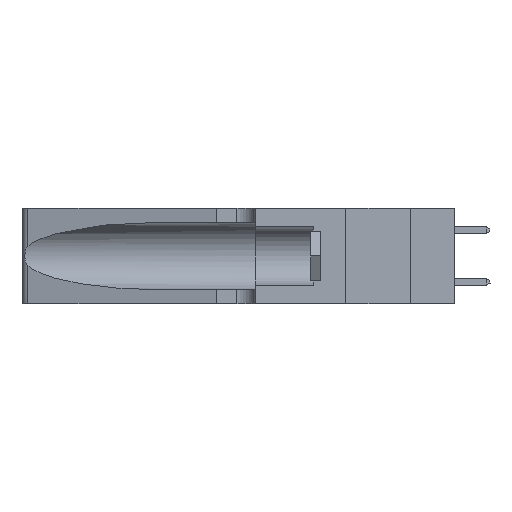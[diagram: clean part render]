
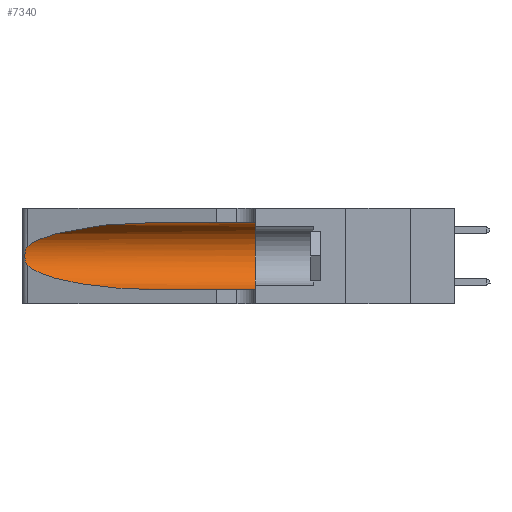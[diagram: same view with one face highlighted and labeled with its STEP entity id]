
A CAD part, left-side view. The second image highlights one B-rep face of the part: STEP entity #7340.
In plain terms, the highlighted cylindrical face has radius 3.308 mm (diameter 6.617 mm), a partial arc.
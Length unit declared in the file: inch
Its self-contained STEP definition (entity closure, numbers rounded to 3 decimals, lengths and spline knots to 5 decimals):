
#622 = CARTESIAN_POINT ( 'NONE',  ( 0.25555, 1.22994, 0.2215 ) ) ;
#775 = CARTESIAN_POINT ( 'NONE',  ( 0.25639, 1.23186, 0.15144 ) ) ;
#1022 = EDGE_CURVE ( 'NONE', #10462, #40487, #26562, .T. ) ;
#1375 = ORIENTED_EDGE ( 'NONE', *, *, #4020, .T. ) ;
#1956 = CARTESIAN_POINT ( 'NONE',  ( 0.2373, 1.15595, 0.28018 ) ) ;
#2164 = CARTESIAN_POINT ( 'NONE',  ( 0.1305, 1.61858, 0.05475 ) ) ;
#3969 = DIRECTION ( 'NONE',  ( 0., 1., 0. ) ) ;
#4020 = EDGE_CURVE ( 'NONE', #10462, #8143, #30314, .T. ) ;
#4248 = CARTESIAN_POINT ( 'NONE',  ( 0.25487, 1.22718, 0.14631 ) ) ;
#4507 = VERTEX_POINT ( 'NONE', #24867 ) ;
#6397 = DIRECTION ( 'NONE',  ( 0., 0., -1. ) ) ;
#6843 = B_SPLINE_CURVE_WITH_KNOTS ( 'NONE', 3,
 ( #24327, #622, #7520, #31050, #10966, #34433, #14373, #37853, #17727, #41245, #21098, #775, #24480, #4248 ),
 .UNSPECIFIED., .F., .F.,
 ( 4, 2, 2, 2, 2, 2, 4 ),
 ( 0., 0.00027, 0.00053, 0.00107, 0.0016, 0.00187, 0.00214 ),
 .UNSPECIFIED. ) ;
#7340 = ADVANCED_FACE ( 'NONE', ( #22718 ), #19573, .F. ) ;
#7520 = CARTESIAN_POINT ( 'NONE',  ( 0.25639, 1.23184, 0.21858 ) ) ;
#8143 = VERTEX_POINT ( 'NONE', #14239 ) ;
#9499 = EDGE_CURVE ( 'NONE', #40487, #18419, #14676, .T. ) ;
#10462 = VERTEX_POINT ( 'NONE', #15334 ) ;
#10966 = CARTESIAN_POINT ( 'NONE',  ( 0.25854, 1.2359, 0.20912 ) ) ;
#11624 = EDGE_CURVE ( 'NONE', #8143, #4507, #6843, .T. ) ;
#12031 = ORIENTED_EDGE ( 'NONE', *, *, #34975, .T. ) ;
#13264 = DIRECTION ( 'NONE',  ( 0., -1., 0. ) ) ;
#14239 = CARTESIAN_POINT ( 'NONE',  ( 0.25487, 1.22718, 0.22369 ) ) ;
#14373 = CARTESIAN_POINT ( 'NONE',  ( 0.26075, 1.23896, 0.19203 ) ) ;
#14380 = CARTESIAN_POINT ( 'NONE',  ( 0.2373, 1.15595, 0.08982 ) ) ;
#14532 = CARTESIAN_POINT ( 'NONE',  ( 0.1305, 0.72297, 0.05475 ) ) ;
#14676 = CIRCLE ( 'NONE', #28606, 0.13025 ) ;
#15184 = ORIENTED_EDGE ( 'NONE', *, *, #1022, .F. ) ;
#15334 = CARTESIAN_POINT ( 'NONE',  ( 0.1305, 0.72297, 0.31525 ) ) ;
#16692 = CARTESIAN_POINT ( 'NONE',  ( 0.1305, 0.72297, 0.05475 ) ) ;
#17308 = CARTESIAN_POINT ( 'NONE',  ( 0.1305, 0.35, 0.31525 ) ) ;
#17727 = CARTESIAN_POINT ( 'NONE',  ( 0.26017, 1.23833, 0.17102 ) ) ;
#18419 = VERTEX_POINT ( 'NONE', #39879 ) ;
#18583 = ORIENTED_EDGE ( 'NONE', *, *, #11624, .T. ) ;
#18884 = CARTESIAN_POINT ( 'NONE',  ( 0.1305, 0.72297, 0.31525 ) ) ;
#19573 = CYLINDRICAL_SURFACE ( 'NONE', #26866, 0.13025 ) ;
#20460 = DIRECTION ( 'NONE',  ( 0., -1., 0. ) ) ;
#21098 = CARTESIAN_POINT ( 'NONE',  ( 0.25789, 1.23486, 0.15765 ) ) ;
#21103 = CARTESIAN_POINT ( 'NONE',  ( 0.25487, 1.22718, 0.14631 ) ) ;
#22250 = CARTESIAN_POINT ( 'NONE',  ( 0.18966, 0.96281, 0.31525 ) ) ;
#22718 = FACE_OUTER_BOUND ( 'NONE', #41800, .T. ) ;
#24195 = CARTESIAN_POINT ( 'NONE',  ( 0.1305, 0.35, 0.185 ) ) ;
#24327 = CARTESIAN_POINT ( 'NONE',  ( 0.25487, 1.22718, 0.22369 ) ) ;
#24480 = CARTESIAN_POINT ( 'NONE',  ( 0.25555, 1.22993, 0.14849 ) ) ;
#24867 = CARTESIAN_POINT ( 'NONE',  ( 0.25487, 1.22718, 0.14631 ) ) ;
#25508 = VECTOR ( 'NONE', #20460, 39.37008 ) ;
#25614 = CARTESIAN_POINT ( 'NONE',  ( 0.25487, 1.22718, 0.22369 ) ) ;
#25801 = DIRECTION ( 'NONE',  ( 0., -1., 0. ) ) ;
#26562 = LINE ( 'NONE', #33798, #25508 ) ;
#26866 = AXIS2_PLACEMENT_3D ( 'NONE', #29937, #13264, #6397 ) ;
#27546 = DIRECTION ( 'NONE',  ( 0., 0., 1. ) ) ;
#27552 = ORIENTED_EDGE ( 'NONE', *, *, #9499, .F. ) ;
#28606 = AXIS2_PLACEMENT_3D ( 'NONE', #24195, #3969, #27546 ) ;
#29937 = CARTESIAN_POINT ( 'NONE',  ( 0.1305, 1.61858, 0.185 ) ) ;
#30314 =( BOUNDED_CURVE ( )  B_SPLINE_CURVE ( 3, ( #18884, #22250, #1956, #25614 ),
 .UNSPECIFIED., .F., .F. ) 
 B_SPLINE_CURVE_WITH_KNOTS ( ( 4, 4 ),
 ( 1.5708, 2.84003 ),
 .UNSPECIFIED. ) 
 CURVE ( )  GEOMETRIC_REPRESENTATION_ITEM ( )  RATIONAL_B_SPLINE_CURVE ( ( 1., 0.87, 0.87, 1. ) ) 
 REPRESENTATION_ITEM ( '' )  );
#30492 = LINE ( 'NONE', #2164, #39482 ) ;
#31050 = CARTESIAN_POINT ( 'NONE',  ( 0.25787, 1.23484, 0.2124 ) ) ;
#31654 =( BOUNDED_CURVE ( )  B_SPLINE_CURVE ( 3, ( #21103, #14380, #34586, #14532 ),
 .UNSPECIFIED., .F., .F. ) 
 B_SPLINE_CURVE_WITH_KNOTS ( ( 4, 4 ),
 ( 3.44316, 4.71239 ),
 .UNSPECIFIED. ) 
 CURVE ( )  GEOMETRIC_REPRESENTATION_ITEM ( )  RATIONAL_B_SPLINE_CURVE ( ( 1., 0.87, 0.87, 1. ) ) 
 REPRESENTATION_ITEM ( '' )  );
#33718 = ORIENTED_EDGE ( 'NONE', *, *, #43360, .T. ) ;
#33798 = CARTESIAN_POINT ( 'NONE',  ( 0.1305, 1.61858, 0.31525 ) ) ;
#34433 = CARTESIAN_POINT ( 'NONE',  ( 0.26018, 1.23835, 0.19895 ) ) ;
#34586 = CARTESIAN_POINT ( 'NONE',  ( 0.18966, 0.96281, 0.05475 ) ) ;
#34975 = EDGE_CURVE ( 'NONE', #38429, #18419, #30492, .T. ) ;
#37853 = CARTESIAN_POINT ( 'NONE',  ( 0.26075, 1.23896, 0.178 ) ) ;
#38429 = VERTEX_POINT ( 'NONE', #16692 ) ;
#39482 = VECTOR ( 'NONE', #25801, 39.37008 ) ;
#39879 = CARTESIAN_POINT ( 'NONE',  ( 0.1305, 0.35, 0.05475 ) ) ;
#40487 = VERTEX_POINT ( 'NONE', #17308 ) ;
#41245 = CARTESIAN_POINT ( 'NONE',  ( 0.25856, 1.23593, 0.16098 ) ) ;
#41800 = EDGE_LOOP ( 'NONE', ( #1375, #18583, #33718, #12031, #27552, #15184 ) ) ;
#43360 = EDGE_CURVE ( 'NONE', #4507, #38429, #31654, .T. ) ;
